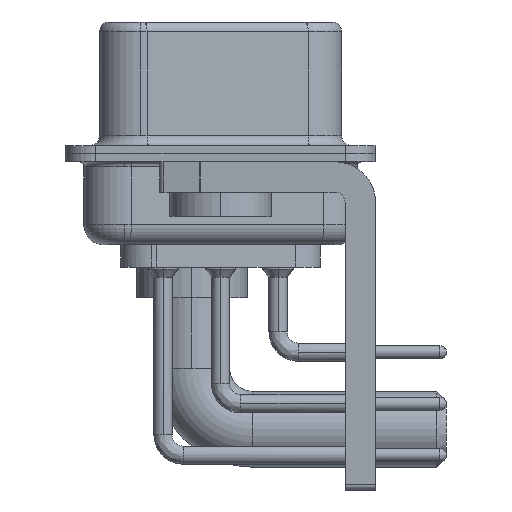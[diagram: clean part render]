
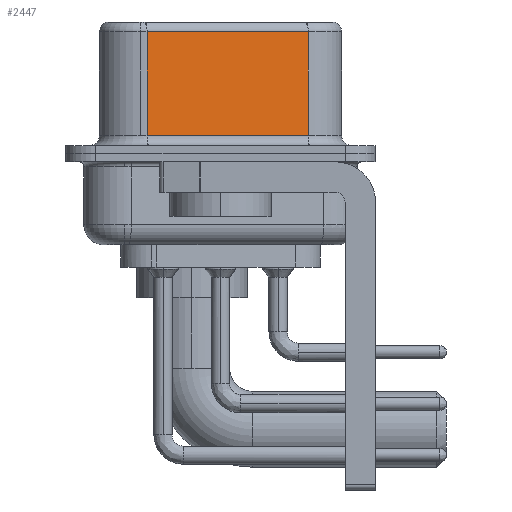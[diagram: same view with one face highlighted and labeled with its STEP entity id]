
A CAD part, left-side view. The second image highlights one B-rep face of the part: STEP entity #2447.
In plain terms, the highlighted planar face has unit normal (-0.985, -0.174, 0).
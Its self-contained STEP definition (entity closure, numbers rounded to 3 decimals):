
#1011 = ORIENTED_EDGE ( 'NONE', *, *, #10740, .F. ) ;
#1028 = CARTESIAN_POINT ( 'NONE',  ( 5.132, -4.322, 0.9 ) ) ;
#2447 = ADVANCED_FACE ( 'NONE', ( #5028 ), #29713, .F. ) ;
#2504 = VECTOR ( 'NONE', #8511, 1000. ) ;
#2949 = VERTEX_POINT ( 'NONE', #16982 ) ;
#3085 = EDGE_CURVE ( 'NONE', #2949, #30099, #11696, .T. ) ;
#3374 = VERTEX_POINT ( 'NONE', #19574 ) ;
#3906 = VECTOR ( 'NONE', #18971, 1000. ) ;
#5028 = FACE_OUTER_BOUND ( 'NONE', #17281, .T. ) ;
#7829 = DIRECTION ( 'NONE',  ( -0.174, 0.985, 0. ) ) ;
#8511 = DIRECTION ( 'NONE',  ( -0.174, 0.985, 0. ) ) ;
#9379 = ORIENTED_EDGE ( 'NONE', *, *, #15477, .T. ) ;
#9571 = CARTESIAN_POINT ( 'NONE',  ( 5.132, -4.322, 6.52 ) ) ;
#9665 = CARTESIAN_POINT ( 'NONE',  ( 3.73, 3.628, 6.02 ) ) ;
#10296 = VECTOR ( 'NONE', #24157, 1000. ) ;
#10740 = EDGE_CURVE ( 'NONE', #2949, #17773, #21598, .T. ) ;
#11696 = LINE ( 'NONE', #23195, #2504 ) ;
#12000 = CARTESIAN_POINT ( 'NONE',  ( 5.132, -4.322, 0.9 ) ) ;
#15477 = EDGE_CURVE ( 'NONE', #3374, #17773, #21038, .T. ) ;
#16982 = CARTESIAN_POINT ( 'NONE',  ( 5.132, -4.322, 6.02 ) ) ;
#17281 = EDGE_LOOP ( 'NONE', ( #1011, #36816, #33493, #9379 ) ) ;
#17773 = VERTEX_POINT ( 'NONE', #1028 ) ;
#18971 = DIRECTION ( 'NONE',  ( 0., 0., -1. ) ) ;
#19574 = CARTESIAN_POINT ( 'NONE',  ( 3.73, 3.628, 0.9 ) ) ;
#21038 = LINE ( 'NONE', #12000, #26901 ) ;
#21598 = LINE ( 'NONE', #33259, #3906 ) ;
#22070 = LINE ( 'NONE', #33556, #10296 ) ;
#23195 = CARTESIAN_POINT ( 'NONE',  ( 5.132, -4.322, 6.02 ) ) ;
#24157 = DIRECTION ( 'NONE',  ( 0., 0., -1. ) ) ;
#24959 = DIRECTION ( 'NONE',  ( 0.985, 0.174, 0. ) ) ;
#25113 = AXIS2_PLACEMENT_3D ( 'NONE', #9571, #24959, #7829 ) ;
#26901 = VECTOR ( 'NONE', #35172, 1000. ) ;
#29713 = PLANE ( 'NONE',  #25113 ) ;
#30099 = VERTEX_POINT ( 'NONE', #9665 ) ;
#33259 = CARTESIAN_POINT ( 'NONE',  ( 5.132, -4.322, 6.52 ) ) ;
#33493 = ORIENTED_EDGE ( 'NONE', *, *, #36178, .T. ) ;
#33556 = CARTESIAN_POINT ( 'NONE',  ( 3.73, 3.628, 6.52 ) ) ;
#35172 = DIRECTION ( 'NONE',  ( 0.174, -0.985, 0. ) ) ;
#36178 = EDGE_CURVE ( 'NONE', #30099, #3374, #22070, .T. ) ;
#36816 = ORIENTED_EDGE ( 'NONE', *, *, #3085, .T. ) ;
